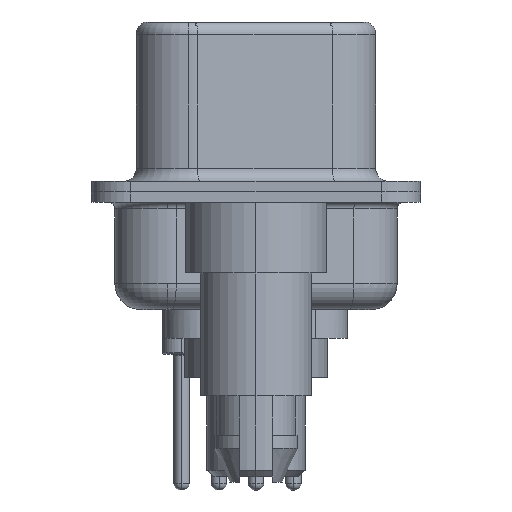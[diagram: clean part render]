
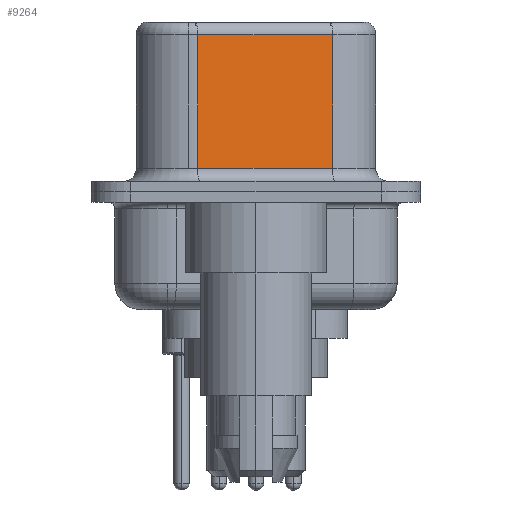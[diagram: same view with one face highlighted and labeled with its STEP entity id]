
A CAD part, left-side view. The second image highlights one B-rep face of the part: STEP entity #9264.
In plain terms, the highlighted planar face has unit normal (-0.985, -0.174, 0).
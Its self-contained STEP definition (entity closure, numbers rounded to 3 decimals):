
#406 = DIRECTION ( 'NONE',  ( 0.985, 0.174, 0. ) ) ;
#411 = CARTESIAN_POINT ( 'NONE',  ( 4.58, -2.927, 6.02 ) ) ;
#843 = CARTESIAN_POINT ( 'NONE',  ( 4.58, -2.927, 6.02 ) ) ;
#915 = LINE ( 'NONE', #843, #1415 ) ;
#1415 = VECTOR ( 'NONE', #12302, 1000. ) ;
#2186 = CARTESIAN_POINT ( 'NONE',  ( 3.67, 2.233, 6.52 ) ) ;
#3480 = VECTOR ( 'NONE', #16453, 1000. ) ;
#3499 = LINE ( 'NONE', #2186, #16028 ) ;
#3747 = CARTESIAN_POINT ( 'NONE',  ( 3.67, 2.233, 6.02 ) ) ;
#4603 = EDGE_LOOP ( 'NONE', ( #6917, #12114, #10495, #20362 ) ) ;
#5002 = CARTESIAN_POINT ( 'NONE',  ( 4.58, -2.927, 6.52 ) ) ;
#5053 = CARTESIAN_POINT ( 'NONE',  ( 4.58, -2.927, 0.9 ) ) ;
#6390 = VECTOR ( 'NONE', #13154, 1000. ) ;
#6897 = LINE ( 'NONE', #5002, #6390 ) ;
#6917 = ORIENTED_EDGE ( 'NONE', *, *, #14443, .F. ) ;
#8284 = VERTEX_POINT ( 'NONE', #14454 ) ;
#8736 = EDGE_CURVE ( 'NONE', #11894, #19164, #915, .T. ) ;
#9264 = ADVANCED_FACE ( 'NONE', ( #18552 ), #11913, .F. ) ;
#10495 = ORIENTED_EDGE ( 'NONE', *, *, #17214, .T. ) ;
#11894 = VERTEX_POINT ( 'NONE', #411 ) ;
#11913 = PLANE ( 'NONE',  #13345 ) ;
#12114 = ORIENTED_EDGE ( 'NONE', *, *, #8736, .T. ) ;
#12302 = DIRECTION ( 'NONE',  ( -0.174, 0.985, 0. ) ) ;
#13154 = DIRECTION ( 'NONE',  ( 0., 0., -1. ) ) ;
#13345 = AXIS2_PLACEMENT_3D ( 'NONE', #20084, #406, #13558 ) ;
#13558 = DIRECTION ( 'NONE',  ( -0.174, 0.985, 0. ) ) ;
#13644 = DIRECTION ( 'NONE',  ( 0., 0., -1. ) ) ;
#13939 = CARTESIAN_POINT ( 'NONE',  ( 3.67, 2.233, 0.9 ) ) ;
#14443 = EDGE_CURVE ( 'NONE', #11894, #8284, #6897, .T. ) ;
#14454 = CARTESIAN_POINT ( 'NONE',  ( 4.58, -2.927, 0.9 ) ) ;
#16028 = VECTOR ( 'NONE', #13644, 1000. ) ;
#16453 = DIRECTION ( 'NONE',  ( 0.174, -0.985, 0. ) ) ;
#16515 = LINE ( 'NONE', #5053, #3480 ) ;
#16698 = VERTEX_POINT ( 'NONE', #13939 ) ;
#17214 = EDGE_CURVE ( 'NONE', #19164, #16698, #3499, .T. ) ;
#17657 = EDGE_CURVE ( 'NONE', #16698, #8284, #16515, .T. ) ;
#18552 = FACE_OUTER_BOUND ( 'NONE', #4603, .T. ) ;
#19164 = VERTEX_POINT ( 'NONE', #3747 ) ;
#20084 = CARTESIAN_POINT ( 'NONE',  ( 4.58, -2.927, 6.52 ) ) ;
#20362 = ORIENTED_EDGE ( 'NONE', *, *, #17657, .T. ) ;
